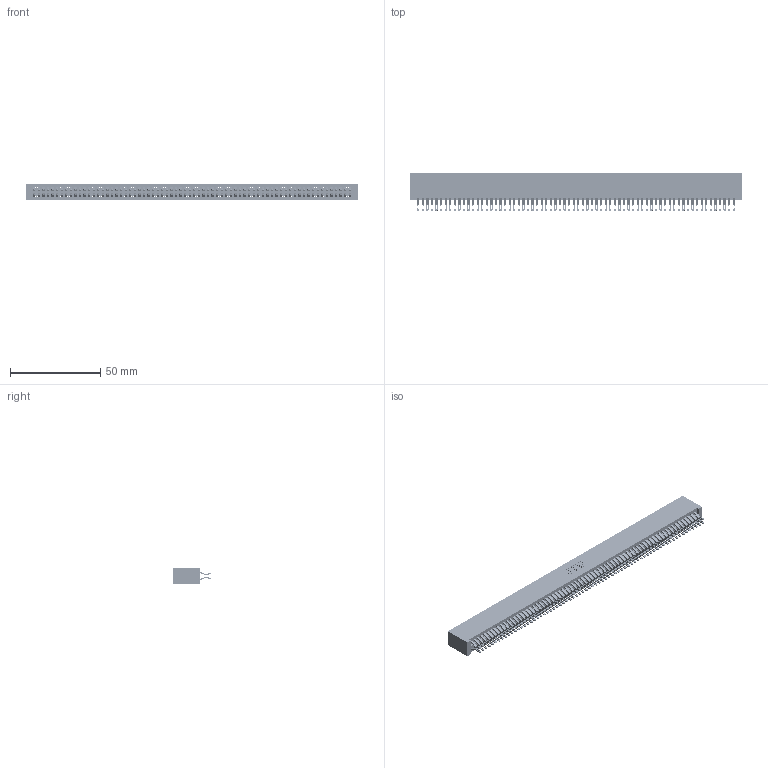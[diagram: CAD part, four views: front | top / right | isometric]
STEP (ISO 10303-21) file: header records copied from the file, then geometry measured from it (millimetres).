
FILE_DESCRIPTION (( 'STEP AP203' ), '1' );
FILE_NAME ('345-140-555-201.STEP', '2018-10-21T00:57:17', ( '' ), ( '' ), 'SwSTEP 2.0', 'SolidWorks 2016', '' );
FILE_SCHEMA (( 'CONFIG_CONTROL_DESIGN' ));
Length unit declared in the file: inch
Products named in the file (3): 345-140-555-201; 345-292-001_555 Tail; 345 Part_No Mounting Lugs
Assembly tree (141 placements, depth 2):
  345-140-555-201
    345 Part_No Mounting Lugs
    345-292-001_555 Tail  x140
Bounding box: 184.4 x 21.13 x 9.4 mm (x, y, z)
Volume: 19195.1 mm3; surface area: 30631.5 mm2
Topology: 141 solids, 141 shells, 7958 faces, 25097 edges, 16730 vertices
Faces by surface type: plane 4416, cylinder 3542
Entity records: 51203 total; most frequent: CARTESIAN_POINT 8590, ORIENTED_EDGE 8494, DIRECTION 7503, EDGE_CURVE 4247, LINE 3823, VECTOR 3823, VERTEX_POINT 2830, AXIS2_PLACEMENT_3D 1840
